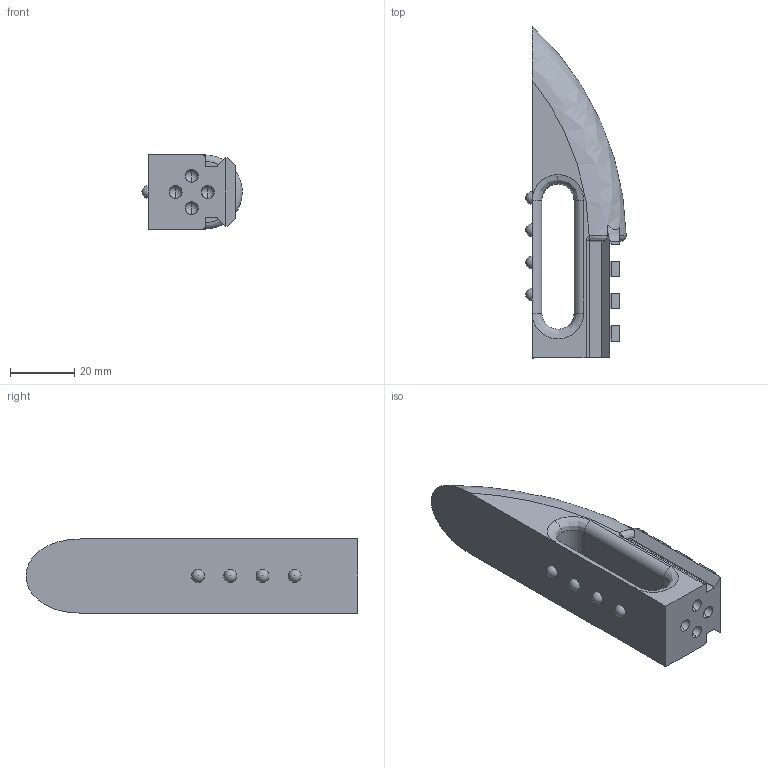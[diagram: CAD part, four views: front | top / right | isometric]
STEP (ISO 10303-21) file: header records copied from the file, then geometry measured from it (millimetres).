
FILE_DESCRIPTION (( 'STEP AP214' ), '1' );
FILE_NAME ('Stock Rail Front.STEP', '2013-06-24T22:49:19', ( 'Asher' ), ( '' ), 'SwSTEP 2.0', 'SolidWorks 2013', '' );
FILE_SCHEMA (( 'AUTOMOTIVE_DESIGN' ));
Length unit declared in the file: millimetre
Products named in the file (1): Stock Rail Front
Bounding box: 31.2 x 103.08 x 23.02 mm (x, y, z)
Volume: 36292.6 mm3; surface area: 11107 mm2
Topology: 1 solids, 1 shells, 80 faces, 238 edges, 152 vertices
Faces by surface type: plane 42, bspline 17, sphere 12, cylinder 9
Entity records: 3246 total; most frequent: CARTESIAN_POINT 1364, ORIENTED_EDGE 416, DIRECTION 334, EDGE_CURVE 208, VERTEX_POINT 136, LINE 120, VECTOR 120, AXIS2_PLACEMENT_3D 107
